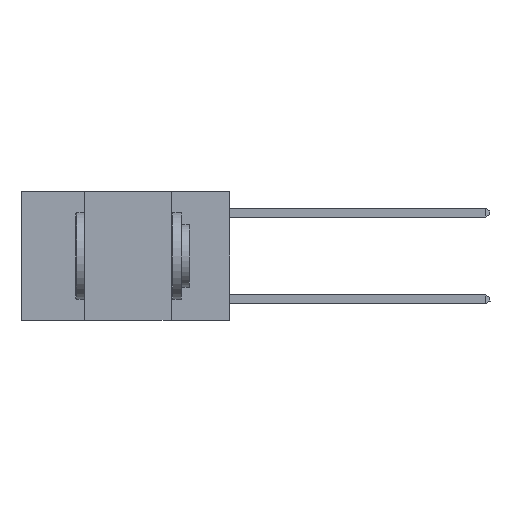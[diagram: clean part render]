
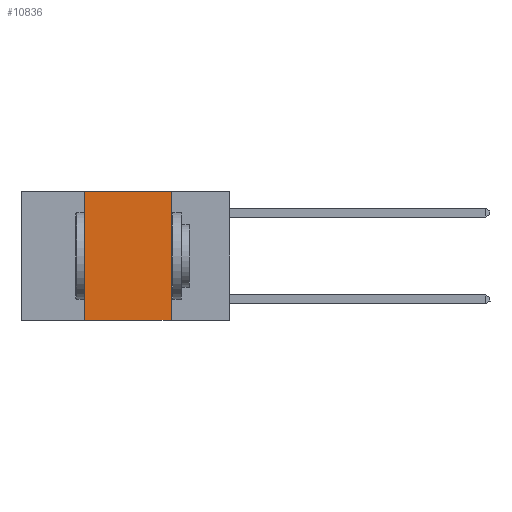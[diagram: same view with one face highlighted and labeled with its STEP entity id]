
A CAD part, left-side view. The second image highlights one B-rep face of the part: STEP entity #10836.
In plain terms, the highlighted planar face has unit normal (-1, 0, 0).
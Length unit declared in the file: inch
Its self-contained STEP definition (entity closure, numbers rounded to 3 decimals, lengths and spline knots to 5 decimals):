
#187 = ORIENTED_EDGE ( 'NONE', *, *, #1502, .F. ) ;
#387 = CARTESIAN_POINT ( 'NONE',  ( 0., 0.17, 0. ) ) ;
#575 = CARTESIAN_POINT ( 'NONE',  ( 0., 0.6, 0. ) ) ;
#1084 = VECTOR ( 'NONE', #2231, 39.37008 ) ;
#1502 = EDGE_CURVE ( 'NONE', #12638, #8776, #1615, .T. ) ;
#1615 = LINE ( 'NONE', #575, #1084 ) ;
#1858 = ORIENTED_EDGE ( 'NONE', *, *, #13379, .F. ) ;
#2231 = DIRECTION ( 'NONE',  ( 0., -1., 0. ) ) ;
#3884 = AXIS2_PLACEMENT_3D ( 'NONE', #11575, #16284, #6908 ) ;
#5319 = PLANE ( 'NONE',  #3884 ) ;
#5573 = CARTESIAN_POINT ( 'NONE',  ( 0., 0.6, -0.37 ) ) ;
#6908 = DIRECTION ( 'NONE',  ( 0., 0., -1. ) ) ;
#7155 = DIRECTION ( 'NONE',  ( 0., -1., 0. ) ) ;
#7638 = CARTESIAN_POINT ( 'NONE',  ( 0., 0.17, 0. ) ) ;
#8326 = LINE ( 'NONE', #17782, #20260 ) ;
#8445 = DIRECTION ( 'NONE',  ( 0., 0., 1. ) ) ;
#8776 = VERTEX_POINT ( 'NONE', #387 ) ;
#9227 = DIRECTION ( 'NONE',  ( 0., 0., -1. ) ) ;
#9386 = FACE_OUTER_BOUND ( 'NONE', #19127, .T. ) ;
#10355 = CARTESIAN_POINT ( 'NONE',  ( 0., 0.17, -0.37 ) ) ;
#10836 = ADVANCED_FACE ( 'NONE', ( #9386 ), #5319, .F. ) ;
#10965 = VERTEX_POINT ( 'NONE', #11221 ) ;
#11221 = CARTESIAN_POINT ( 'NONE',  ( 0., 0.42, -0.37 ) ) ;
#11251 = EDGE_CURVE ( 'NONE', #10965, #18706, #14014, .T. ) ;
#11340 = ORIENTED_EDGE ( 'NONE', *, *, #12304, .F. ) ;
#11575 = CARTESIAN_POINT ( 'NONE',  ( 0., 0.6, 0. ) ) ;
#12304 = EDGE_CURVE ( 'NONE', #10965, #12638, #8326, .T. ) ;
#12638 = VERTEX_POINT ( 'NONE', #15399 ) ;
#13379 = EDGE_CURVE ( 'NONE', #8776, #18706, #15234, .T. ) ;
#14014 = LINE ( 'NONE', #5573, #14514 ) ;
#14514 = VECTOR ( 'NONE', #7155, 39.37008 ) ;
#14754 = VECTOR ( 'NONE', #9227, 39.37008 ) ;
#15234 = LINE ( 'NONE', #7638, #14754 ) ;
#15399 = CARTESIAN_POINT ( 'NONE',  ( 0., 0.42, 0. ) ) ;
#15554 = ORIENTED_EDGE ( 'NONE', *, *, #11251, .T. ) ;
#16284 = DIRECTION ( 'NONE',  ( 1., 0., 0. ) ) ;
#17782 = CARTESIAN_POINT ( 'NONE',  ( 0., 0.42, 0. ) ) ;
#18706 = VERTEX_POINT ( 'NONE', #10355 ) ;
#19127 = EDGE_LOOP ( 'NONE', ( #1858, #187, #11340, #15554 ) ) ;
#20260 = VECTOR ( 'NONE', #8445, 39.37008 ) ;
